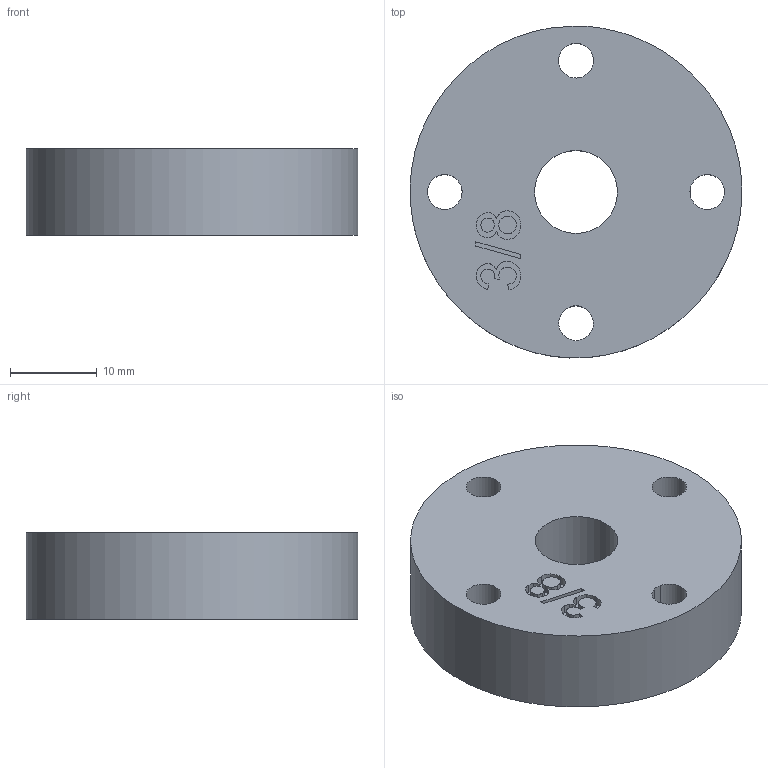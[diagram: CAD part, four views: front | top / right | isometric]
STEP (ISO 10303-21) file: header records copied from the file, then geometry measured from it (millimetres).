
FILE_DESCRIPTION(/* description */ (''),/* implementation_level */ '2;1');
FILE_NAME(/* name */ '8 v2.step',/* time_stamp */ '2022-08-27T22:33:07-04:00',/* author */ (''),/* organization */ (''),/* preprocessor_version */ 'ST-DEVELOPER v19',/* originating_system */ 'Autodesk Translation Framework v11.7.0.108',/* authorisation */ '');
FILE_SCHEMA (('AUTOMOTIVE_DESIGN { 1 0 10303 214 3 1 1 }'));
Length unit declared in the file: millimetre
Products named in the file (1): HiLo JIG_drill guide 3/8
Bounding box: 38.23 x 38.24 x 10 mm (x, y, z)
Volume: 10219.9 mm3; surface area: 4111.6 mm2
Topology: 1 solids, 1 shells, 81 faces, 222 edges, 148 vertices
Faces by surface type: bspline 61, plane 14, cylinder 6
Full cylindrical faces by diameter (mm): 4 x3, 9.55 x1
Entity records: 3268 total; most frequent: CARTESIAN_POINT 1569, ORIENTED_EDGE 444, EDGE_CURVE 222, DIRECTION 154, VERTEX_POINT 148, B_SPLINE_CURVE_WITH_KNOTS 120, EDGE_LOOP 96, LINE 88
